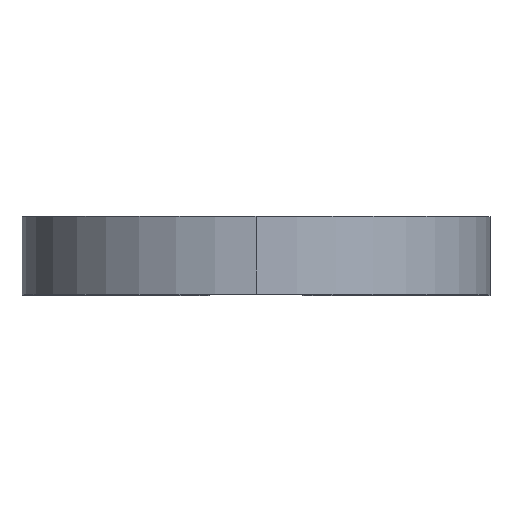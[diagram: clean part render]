
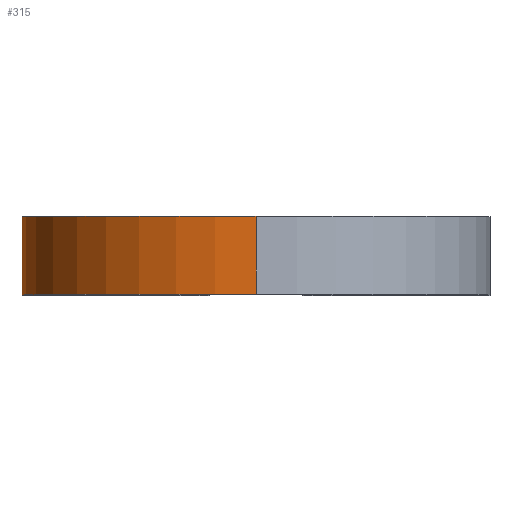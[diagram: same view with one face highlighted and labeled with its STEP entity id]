
A CAD part, top view. The second image highlights one B-rep face of the part: STEP entity #315.
In plain terms, the highlighted cylindrical face has radius 15 mm (diameter 30 mm), a partial arc.
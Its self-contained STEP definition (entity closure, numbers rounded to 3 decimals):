
#23 = DIRECTION ( 'NONE',  ( 0., 1., 0. ) ) ;
#79 = CARTESIAN_POINT ( 'NONE',  ( -14.29, -0.457, 0. ) ) ;
#97 = CARTESIAN_POINT ( 'NONE',  ( -29.29, -0.457, 0. ) ) ;
#100 = CIRCLE ( 'NONE', #885, 15. ) ;
#105 = LINE ( 'NONE', #1382, #789 ) ;
#174 = VERTEX_POINT ( 'NONE', #1223 ) ;
#315 = ADVANCED_FACE ( 'NONE', ( #764 ), #533, .T. ) ;
#350 = ORIENTED_EDGE ( 'NONE', *, *, #1490, .F. ) ;
#380 = VECTOR ( 'NONE', #815, 1000. ) ;
#388 = CARTESIAN_POINT ( 'NONE',  ( -14.29, 4.543, 0. ) ) ;
#417 = AXIS2_PLACEMENT_3D ( 'NONE', #388, #1369, #523 ) ;
#523 = DIRECTION ( 'NONE',  ( 0., 0., -1. ) ) ;
#533 = CYLINDRICAL_SURFACE ( 'NONE', #1643, 15. ) ;
#589 = ORIENTED_EDGE ( 'NONE', *, *, #1563, .T. ) ;
#612 = EDGE_LOOP ( 'NONE', ( #589, #1499, #350, #1601 ) ) ;
#635 = DIRECTION ( 'NONE',  ( 0., 0., 1. ) ) ;
#668 = CARTESIAN_POINT ( 'NONE',  ( -14.29, -0.457, 15. ) ) ;
#761 = LINE ( 'NONE', #992, #380 ) ;
#764 = FACE_OUTER_BOUND ( 'NONE', #612, .T. ) ;
#769 = CARTESIAN_POINT ( 'NONE',  ( -14.29, 4.543, 15. ) ) ;
#789 = VECTOR ( 'NONE', #1424, 1000. ) ;
#815 = DIRECTION ( 'NONE',  ( 0., -1., 0. ) ) ;
#882 = VERTEX_POINT ( 'NONE', #769 ) ;
#885 = AXIS2_PLACEMENT_3D ( 'NONE', #79, #897, #1321 ) ;
#897 = DIRECTION ( 'NONE',  ( 0., -1., 0. ) ) ;
#992 = CARTESIAN_POINT ( 'NONE',  ( -29.29, 4.543, 0. ) ) ;
#1007 = CARTESIAN_POINT ( 'NONE',  ( -14.29, 0., 0. ) ) ;
#1124 = CIRCLE ( 'NONE', #417, 15. ) ;
#1223 = CARTESIAN_POINT ( 'NONE',  ( -29.29, 4.543, 0. ) ) ;
#1267 = EDGE_CURVE ( 'NONE', #1771, #1592, #100, .T. ) ;
#1321 = DIRECTION ( 'NONE',  ( 0., 0., 1. ) ) ;
#1369 = DIRECTION ( 'NONE',  ( 0., 1., 0. ) ) ;
#1382 = CARTESIAN_POINT ( 'NONE',  ( -14.29, -0.457, 15. ) ) ;
#1424 = DIRECTION ( 'NONE',  ( 0., -1., 0. ) ) ;
#1490 = EDGE_CURVE ( 'NONE', #882, #1771, #105, .T. ) ;
#1499 = ORIENTED_EDGE ( 'NONE', *, *, #1267, .F. ) ;
#1563 = EDGE_CURVE ( 'NONE', #174, #1592, #761, .T. ) ;
#1592 = VERTEX_POINT ( 'NONE', #97 ) ;
#1601 = ORIENTED_EDGE ( 'NONE', *, *, #1760, .F. ) ;
#1643 = AXIS2_PLACEMENT_3D ( 'NONE', #1007, #23, #635 ) ;
#1760 = EDGE_CURVE ( 'NONE', #174, #882, #1124, .T. ) ;
#1771 = VERTEX_POINT ( 'NONE', #668 ) ;
